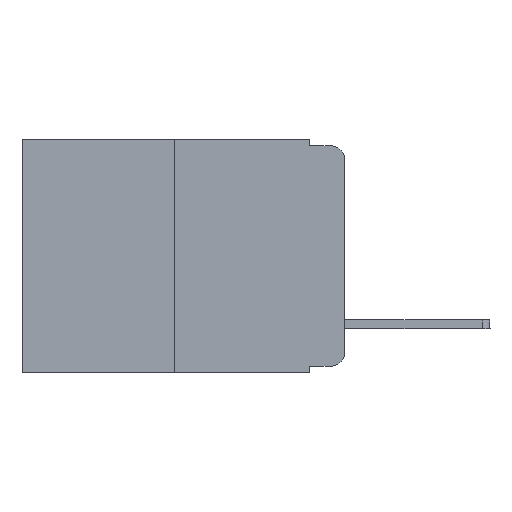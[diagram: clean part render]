
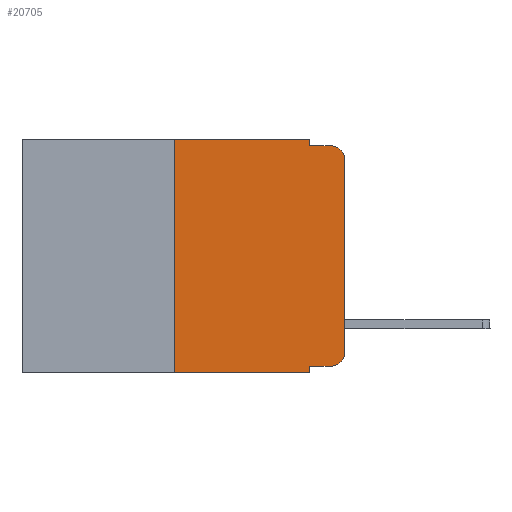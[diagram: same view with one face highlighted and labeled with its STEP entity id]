
A CAD part, left-side view. The second image highlights one B-rep face of the part: STEP entity #20705.
In plain terms, the highlighted planar face has unit normal (-1, 0, 0).
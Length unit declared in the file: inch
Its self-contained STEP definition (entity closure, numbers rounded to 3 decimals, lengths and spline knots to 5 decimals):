
#10 = CIRCLE ( 'NONE', #11872, 0.02 ) ;
#53 = EDGE_CURVE ( 'NONE', #19066, #23062, #23851, .T. ) ;
#120 = CARTESIAN_POINT ( 'NONE',  ( 0., 0.051, 0. ) ) ;
#247 = CARTESIAN_POINT ( 'NONE',  ( 0., 0., -0.03 ) ) ;
#261 = CARTESIAN_POINT ( 'NONE',  ( 0., 0.051, -0.01 ) ) ;
#407 = CARTESIAN_POINT ( 'NONE',  ( 0., 0.02, -0.313 ) ) ;
#600 = LINE ( 'NONE', #19220, #18726 ) ;
#832 = CARTESIAN_POINT ( 'NONE',  ( 0., 0.051, 0. ) ) ;
#1517 = LINE ( 'NONE', #15386, #21137 ) ;
#1821 = EDGE_CURVE ( 'NONE', #6230, #14319, #16286, .T. ) ;
#2433 = DIRECTION ( 'NONE',  ( -1., 0., 0. ) ) ;
#2435 = CARTESIAN_POINT ( 'NONE',  ( 0., 0.051, -0.333 ) ) ;
#2467 = VERTEX_POINT ( 'NONE', #2435 ) ;
#2839 = VERTEX_POINT ( 'NONE', #12928 ) ;
#2927 = EDGE_CURVE ( 'NONE', #2467, #4461, #18595, .T. ) ;
#2949 = CARTESIAN_POINT ( 'NONE',  ( 0., 0.051, -0.343 ) ) ;
#3247 = VECTOR ( 'NONE', #9399, 39.37008 ) ;
#3372 = CARTESIAN_POINT ( 'NONE',  ( 0., 0.473, 0. ) ) ;
#3384 = CARTESIAN_POINT ( 'NONE',  ( 0., 0.02, -0.01 ) ) ;
#3795 = CARTESIAN_POINT ( 'NONE',  ( 0., 0.051, -0.01 ) ) ;
#3899 = CARTESIAN_POINT ( 'NONE',  ( 0., 0.473, -0.343 ) ) ;
#4461 = VERTEX_POINT ( 'NONE', #2949 ) ;
#5349 = DIRECTION ( 'NONE',  ( 1., 0., 0. ) ) ;
#5768 = ORIENTED_EDGE ( 'NONE', *, *, #53, .T. ) ;
#6145 = ORIENTED_EDGE ( 'NONE', *, *, #1821, .F. ) ;
#6230 = VERTEX_POINT ( 'NONE', #23894 ) ;
#6332 = EDGE_CURVE ( 'NONE', #2467, #8749, #20040, .T. ) ;
#8241 = CARTESIAN_POINT ( 'NONE',  ( 0., 0.02, -0.03 ) ) ;
#8749 = VERTEX_POINT ( 'NONE', #9998 ) ;
#9219 = PLANE ( 'NONE',  #11410 ) ;
#9399 = DIRECTION ( 'NONE',  ( 0., 0., -1. ) ) ;
#9438 = VECTOR ( 'NONE', #17069, 39.37008 ) ;
#9565 = ORIENTED_EDGE ( 'NONE', *, *, #19899, .T. ) ;
#9818 = ORIENTED_EDGE ( 'NONE', *, *, #16336, .T. ) ;
#9918 = DIRECTION ( 'NONE',  ( -1., 0., 0. ) ) ;
#9998 = CARTESIAN_POINT ( 'NONE',  ( 0., 0.02, -0.333 ) ) ;
#10893 = ORIENTED_EDGE ( 'NONE', *, *, #19269, .F. ) ;
#11173 = VECTOR ( 'NONE', #12272, 39.37008 ) ;
#11194 = AXIS2_PLACEMENT_3D ( 'NONE', #8241, #9918, #15625 ) ;
#11410 = AXIS2_PLACEMENT_3D ( 'NONE', #3372, #5349, #22564 ) ;
#11563 = CIRCLE ( 'NONE', #11194, 0.02 ) ;
#11710 = VECTOR ( 'NONE', #22815, 39.37008 ) ;
#11872 = AXIS2_PLACEMENT_3D ( 'NONE', #407, #2433, #19183 ) ;
#11988 = DIRECTION ( 'NONE',  ( 0., -1., 0. ) ) ;
#12272 = DIRECTION ( 'NONE',  ( 0., 0., -1. ) ) ;
#12712 = CARTESIAN_POINT ( 'NONE',  ( 0., 0., -0.313 ) ) ;
#12928 = CARTESIAN_POINT ( 'NONE',  ( 0., 0.25, 0. ) ) ;
#13014 = EDGE_CURVE ( 'NONE', #14319, #15341, #13758, .T. ) ;
#13758 = LINE ( 'NONE', #261, #15553 ) ;
#14319 = VERTEX_POINT ( 'NONE', #3795 ) ;
#14678 = ORIENTED_EDGE ( 'NONE', *, *, #2927, .F. ) ;
#15207 = ORIENTED_EDGE ( 'NONE', *, *, #6332, .T. ) ;
#15246 = ORIENTED_EDGE ( 'NONE', *, *, #13014, .F. ) ;
#15341 = VERTEX_POINT ( 'NONE', #3384 ) ;
#15386 = CARTESIAN_POINT ( 'NONE',  ( 0., 0.473, 0. ) ) ;
#15433 = EDGE_CURVE ( 'NONE', #2839, #6230, #1517, .T. ) ;
#15553 = VECTOR ( 'NONE', #19033, 39.37008 ) ;
#15603 = CARTESIAN_POINT ( 'NONE',  ( 0., 0., 0. ) ) ;
#15625 = DIRECTION ( 'NONE',  ( 0., 0., -1. ) ) ;
#16286 = LINE ( 'NONE', #120, #3247 ) ;
#16336 = EDGE_CURVE ( 'NONE', #23062, #15341, #11563, .T. ) ;
#16946 = CARTESIAN_POINT ( 'NONE',  ( 0., 0.051, -0.333 ) ) ;
#17069 = DIRECTION ( 'NONE',  ( 0., -1., 0. ) ) ;
#17432 = CARTESIAN_POINT ( 'NONE',  ( 0., 0.25, -0.343 ) ) ;
#17926 = ORIENTED_EDGE ( 'NONE', *, *, #21209, .T. ) ;
#18595 = LINE ( 'NONE', #832, #11173 ) ;
#18726 = VECTOR ( 'NONE', #23154, 39.37008 ) ;
#18994 = FACE_OUTER_BOUND ( 'NONE', #21478, .T. ) ;
#19033 = DIRECTION ( 'NONE',  ( 0., -1., 0. ) ) ;
#19066 = VERTEX_POINT ( 'NONE', #12712 ) ;
#19183 = DIRECTION ( 'NONE',  ( 0., 0., -1. ) ) ;
#19220 = CARTESIAN_POINT ( 'NONE',  ( 0., 0.25, 0. ) ) ;
#19269 = EDGE_CURVE ( 'NONE', #24173, #2839, #600, .T. ) ;
#19290 = DIRECTION ( 'NONE',  ( 0., 0., 1. ) ) ;
#19591 = LINE ( 'NONE', #3899, #9438 ) ;
#19899 = EDGE_CURVE ( 'NONE', #8749, #19066, #10, .T. ) ;
#20040 = LINE ( 'NONE', #16946, #11710 ) ;
#20705 = ADVANCED_FACE ( 'NONE', ( #18994 ), #9219, .F. ) ;
#21137 = VECTOR ( 'NONE', #11988, 39.37008 ) ;
#21209 = EDGE_CURVE ( 'NONE', #24173, #4461, #19591, .T. ) ;
#21478 = EDGE_LOOP ( 'NONE', ( #5768, #9818, #15246, #6145, #21910, #10893, #17926, #14678, #15207, #9565 ) ) ;
#21910 = ORIENTED_EDGE ( 'NONE', *, *, #15433, .F. ) ;
#22564 = DIRECTION ( 'NONE',  ( 0., 0., -1. ) ) ;
#22815 = DIRECTION ( 'NONE',  ( 0., -1., 0. ) ) ;
#23062 = VERTEX_POINT ( 'NONE', #247 ) ;
#23154 = DIRECTION ( 'NONE',  ( 0., 0., 1. ) ) ;
#23851 = LINE ( 'NONE', #15603, #24446 ) ;
#23894 = CARTESIAN_POINT ( 'NONE',  ( 0., 0.051, 0. ) ) ;
#24173 = VERTEX_POINT ( 'NONE', #17432 ) ;
#24446 = VECTOR ( 'NONE', #19290, 39.37008 ) ;
